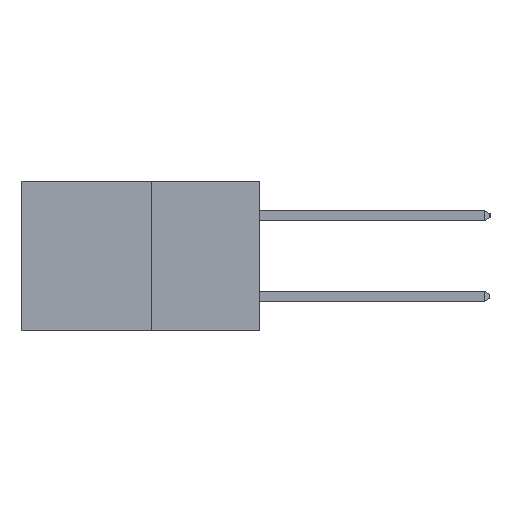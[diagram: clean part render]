
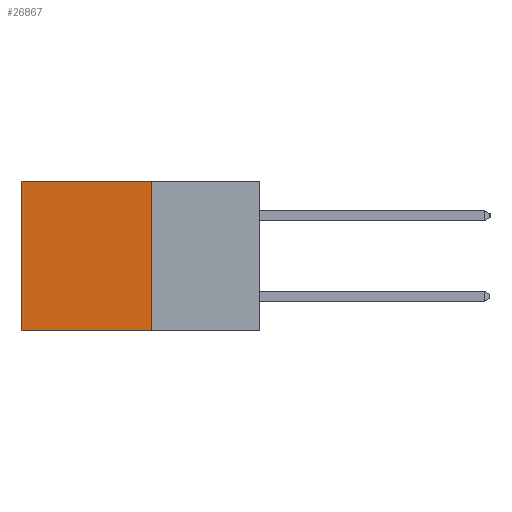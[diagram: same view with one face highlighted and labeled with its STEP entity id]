
A CAD part, left-side view. The second image highlights one B-rep face of the part: STEP entity #26867.
In plain terms, the highlighted planar face has unit normal (-1, 0, 0).
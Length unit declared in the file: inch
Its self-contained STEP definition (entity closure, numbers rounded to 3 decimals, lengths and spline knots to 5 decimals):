
#174 = CARTESIAN_POINT ( 'NONE',  ( 0.277, 0.59, -0.37 ) ) ;
#1678 = AXIS2_PLACEMENT_3D ( 'NONE', #26260, #28704, #14704 ) ;
#1741 = EDGE_CURVE ( 'NONE', #27223, #16891, #19841, .T. ) ;
#3219 = VECTOR ( 'NONE', #30301, 39.37008 ) ;
#3482 = VERTEX_POINT ( 'NONE', #26369 ) ;
#4033 = ORIENTED_EDGE ( 'NONE', *, *, #1741, .F. ) ;
#4230 = EDGE_LOOP ( 'NONE', ( #16442, #4033, #19896, #25364 ) ) ;
#7500 = CARTESIAN_POINT ( 'NONE',  ( 0.277, 0.27, -0.37 ) ) ;
#11273 = FACE_OUTER_BOUND ( 'NONE', #4230, .T. ) ;
#11620 = CARTESIAN_POINT ( 'NONE',  ( 0.277, 0.27, 0. ) ) ;
#12336 = PLANE ( 'NONE',  #1678 ) ;
#12758 = LINE ( 'NONE', #174, #29934 ) ;
#14684 = DIRECTION ( 'NONE',  ( 0., 0., -1. ) ) ;
#14704 = DIRECTION ( 'NONE',  ( 0., 0., -1. ) ) ;
#16442 = ORIENTED_EDGE ( 'NONE', *, *, #26822, .T. ) ;
#16891 = VERTEX_POINT ( 'NONE', #22899 ) ;
#19029 = LINE ( 'NONE', #7500, #24489 ) ;
#19241 = DIRECTION ( 'NONE',  ( 0., 0., -1. ) ) ;
#19268 = EDGE_CURVE ( 'NONE', #3482, #27223, #19029, .T. ) ;
#19841 = LINE ( 'NONE', #22561, #25306 ) ;
#19896 = ORIENTED_EDGE ( 'NONE', *, *, #19268, .F. ) ;
#20648 = VERTEX_POINT ( 'NONE', #26586 ) ;
#22177 = LINE ( 'NONE', #11620, #3219 ) ;
#22490 = DIRECTION ( 'NONE',  ( 0., 1., 0. ) ) ;
#22561 = CARTESIAN_POINT ( 'NONE',  ( 0.277, 0.27, -0.37 ) ) ;
#22899 = CARTESIAN_POINT ( 'NONE',  ( 0.277, 0.59, -0.37 ) ) ;
#23848 = EDGE_CURVE ( 'NONE', #3482, #20648, #22177, .T. ) ;
#24489 = VECTOR ( 'NONE', #14684, 39.37008 ) ;
#25091 = CARTESIAN_POINT ( 'NONE',  ( 0.277, 0.27, -0.37 ) ) ;
#25306 = VECTOR ( 'NONE', #22490, 39.37008 ) ;
#25364 = ORIENTED_EDGE ( 'NONE', *, *, #23848, .T. ) ;
#26260 = CARTESIAN_POINT ( 'NONE',  ( 0.277, 0.27, -0.37 ) ) ;
#26369 = CARTESIAN_POINT ( 'NONE',  ( 0.277, 0.27, 0. ) ) ;
#26586 = CARTESIAN_POINT ( 'NONE',  ( 0.277, 0.59, 0. ) ) ;
#26822 = EDGE_CURVE ( 'NONE', #20648, #16891, #12758, .T. ) ;
#26867 = ADVANCED_FACE ( 'NONE', ( #11273 ), #12336, .F. ) ;
#27223 = VERTEX_POINT ( 'NONE', #25091 ) ;
#28704 = DIRECTION ( 'NONE',  ( 1., 0., 0. ) ) ;
#29934 = VECTOR ( 'NONE', #19241, 39.37008 ) ;
#30301 = DIRECTION ( 'NONE',  ( 0., 1., 0. ) ) ;
